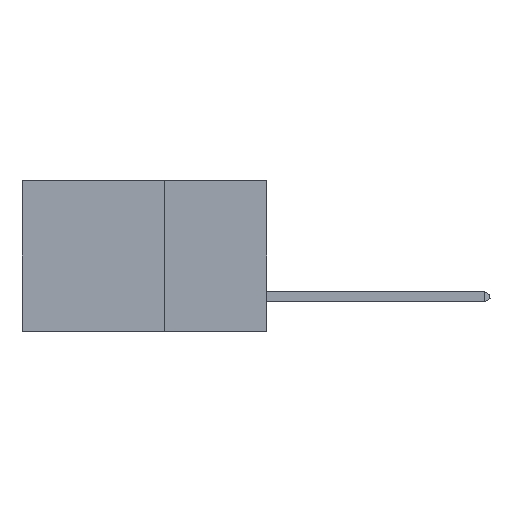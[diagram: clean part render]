
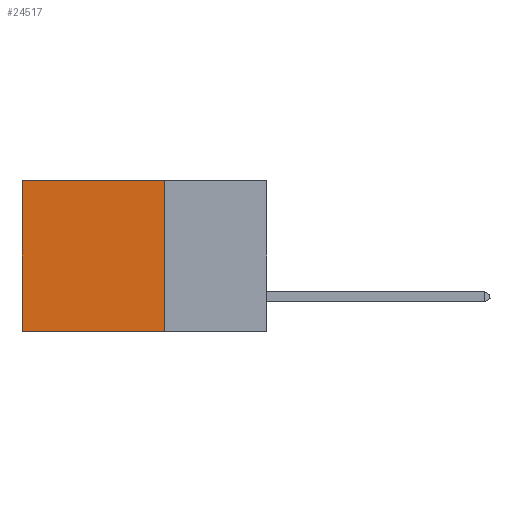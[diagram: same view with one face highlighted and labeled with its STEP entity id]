
A CAD part, left-side view. The second image highlights one B-rep face of the part: STEP entity #24517.
In plain terms, the highlighted planar face has unit normal (-1, 0, 0).
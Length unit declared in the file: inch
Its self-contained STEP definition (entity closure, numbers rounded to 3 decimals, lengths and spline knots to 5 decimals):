
#113 = LINE ( 'NONE', #18057, #13317 ) ;
#919 = CARTESIAN_POINT ( 'NONE',  ( 0.2875, 0.6, 0. ) ) ;
#2171 = DIRECTION ( 'NONE',  ( 0., 1., 0. ) ) ;
#2808 = VERTEX_POINT ( 'NONE', #5247 ) ;
#3212 = DIRECTION ( 'NONE',  ( 0., 0., -1. ) ) ;
#3587 = LINE ( 'NONE', #17137, #19339 ) ;
#3973 = EDGE_CURVE ( 'NONE', #9927, #12613, #4653, .T. ) ;
#4653 = LINE ( 'NONE', #7990, #6200 ) ;
#5247 = CARTESIAN_POINT ( 'NONE',  ( 0.2875, 0.6, -0.37 ) ) ;
#6200 = VECTOR ( 'NONE', #2171, 39.37008 ) ;
#6241 = DIRECTION ( 'NONE',  ( 0., 1., 0. ) ) ;
#7990 = CARTESIAN_POINT ( 'NONE',  ( 0.2875, 0.25, 0. ) ) ;
#9927 = VERTEX_POINT ( 'NONE', #18811 ) ;
#10843 = CARTESIAN_POINT ( 'NONE',  ( 0.2875, 0.6, 0. ) ) ;
#11135 = CARTESIAN_POINT ( 'NONE',  ( 0.2875, 0.25, 0. ) ) ;
#11596 = VECTOR ( 'NONE', #15001, 39.37008 ) ;
#12613 = VERTEX_POINT ( 'NONE', #10843 ) ;
#13158 = DIRECTION ( 'NONE',  ( 0., 0., -1. ) ) ;
#13317 = VECTOR ( 'NONE', #6241, 39.37008 ) ;
#15001 = DIRECTION ( 'NONE',  ( 0., 0., -1. ) ) ;
#16840 = ORIENTED_EDGE ( 'NONE', *, *, #17017, .F. ) ;
#17017 = EDGE_CURVE ( 'NONE', #9927, #17907, #3587, .T. ) ;
#17137 = CARTESIAN_POINT ( 'NONE',  ( 0.2875, 0.25, 0. ) ) ;
#17907 = VERTEX_POINT ( 'NONE', #20828 ) ;
#18057 = CARTESIAN_POINT ( 'NONE',  ( 0.2875, 0.25, -0.37 ) ) ;
#18069 = FACE_OUTER_BOUND ( 'NONE', #20779, .T. ) ;
#18811 = CARTESIAN_POINT ( 'NONE',  ( 0.2875, 0.25, 0. ) ) ;
#18838 = ORIENTED_EDGE ( 'NONE', *, *, #19603, .F. ) ;
#19148 = PLANE ( 'NONE',  #20678 ) ;
#19339 = VECTOR ( 'NONE', #13158, 39.37008 ) ;
#19603 = EDGE_CURVE ( 'NONE', #17907, #2808, #113, .T. ) ;
#20678 = AXIS2_PLACEMENT_3D ( 'NONE', #11135, #24897, #3212 ) ;
#20779 = EDGE_LOOP ( 'NONE', ( #22714, #18838, #16840, #22003 ) ) ;
#20828 = CARTESIAN_POINT ( 'NONE',  ( 0.2875, 0.25, -0.37 ) ) ;
#22003 = ORIENTED_EDGE ( 'NONE', *, *, #3973, .T. ) ;
#22387 = LINE ( 'NONE', #919, #11596 ) ;
#22714 = ORIENTED_EDGE ( 'NONE', *, *, #23675, .T. ) ;
#23675 = EDGE_CURVE ( 'NONE', #12613, #2808, #22387, .T. ) ;
#24517 = ADVANCED_FACE ( 'NONE', ( #18069 ), #19148, .F. ) ;
#24897 = DIRECTION ( 'NONE',  ( 1., 0., 0. ) ) ;
